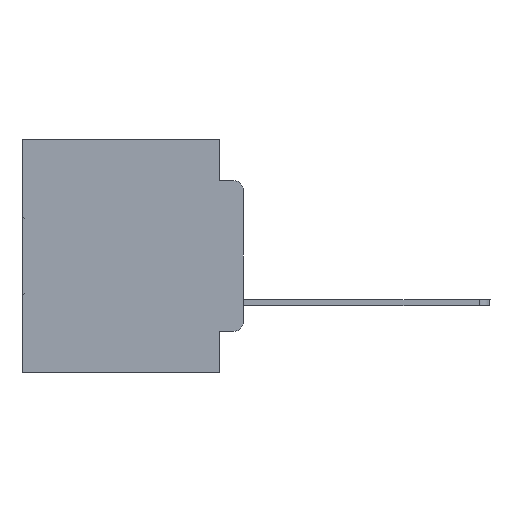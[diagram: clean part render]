
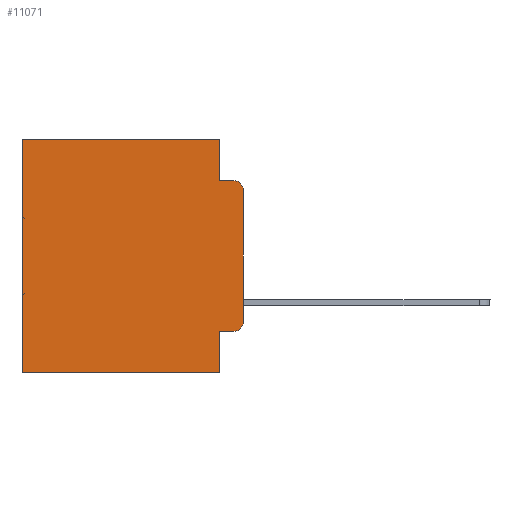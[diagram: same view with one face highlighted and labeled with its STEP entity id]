
A CAD part, left-side view. The second image highlights one B-rep face of the part: STEP entity #11071.
In plain terms, the highlighted planar face has unit normal (-1, 0, 0).
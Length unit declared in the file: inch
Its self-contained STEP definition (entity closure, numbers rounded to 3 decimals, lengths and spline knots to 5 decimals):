
#375 = CARTESIAN_POINT ( 'NONE',  ( 0.298, 0., 0. ) ) ;
#809 = CARTESIAN_POINT ( 'NONE',  ( 0.298, 0.473, 0. ) ) ;
#966 = VECTOR ( 'NONE', #11228, 39.37008 ) ;
#1144 = VERTEX_POINT ( 'NONE', #7849 ) ;
#1548 = EDGE_LOOP ( 'NONE', ( #2685, #17190, #29655, #28987, #21260, #29517, #4103, #18307, #16381, #31728 ) ) ;
#1833 = CARTESIAN_POINT ( 'NONE',  ( 0.298, 0.473, 0. ) ) ;
#1948 = LINE ( 'NONE', #13682, #32490 ) ;
#2402 = CARTESIAN_POINT ( 'NONE',  ( 0.298, 0.051, -0.4115 ) ) ;
#2685 = ORIENTED_EDGE ( 'NONE', *, *, #7705, .F. ) ;
#4091 = DIRECTION ( 'NONE',  ( -1., 0., 0. ) ) ;
#4103 = ORIENTED_EDGE ( 'NONE', *, *, #4304, .F. ) ;
#4304 = EDGE_CURVE ( 'NONE', #33011, #7289, #14189, .T. ) ;
#4448 = DIRECTION ( 'NONE',  ( 0., 0., -1. ) ) ;
#5104 = CARTESIAN_POINT ( 'NONE',  ( 0.298, 0.02, -0.3915 ) ) ;
#5167 = VERTEX_POINT ( 'NONE', #2402 ) ;
#5868 = EDGE_CURVE ( 'NONE', #33396, #25207, #22810, .T. ) ;
#6912 = CARTESIAN_POINT ( 'NONE',  ( 0.298, 0.02, -0.0885 ) ) ;
#7289 = VERTEX_POINT ( 'NONE', #31717 ) ;
#7705 = EDGE_CURVE ( 'NONE', #26355, #1144, #12773, .T. ) ;
#7849 = CARTESIAN_POINT ( 'NONE',  ( 0.298, 0., -0.3915 ) ) ;
#8508 = CARTESIAN_POINT ( 'NONE',  ( 0.298, 0., -0.1085 ) ) ;
#8758 = EDGE_CURVE ( 'NONE', #5167, #13979, #1948, .T. ) ;
#9283 = LINE ( 'NONE', #809, #966 ) ;
#9315 = AXIS2_PLACEMENT_3D ( 'NONE', #5104, #31839, #21213 ) ;
#9506 = CARTESIAN_POINT ( 'NONE',  ( 0.298, 0.051, -0.5 ) ) ;
#9947 = AXIS2_PLACEMENT_3D ( 'NONE', #23318, #17762, #4448 ) ;
#11071 = ADVANCED_FACE ( 'NONE', ( #30177 ), #20005, .F. ) ;
#11228 = DIRECTION ( 'NONE',  ( 0., 0., -1. ) ) ;
#11705 = LINE ( 'NONE', #25382, #27233 ) ;
#11950 = VECTOR ( 'NONE', #20858, 39.37008 ) ;
#12652 = CARTESIAN_POINT ( 'NONE',  ( 0.298, 0., -0.5 ) ) ;
#12773 = LINE ( 'NONE', #15342, #11950 ) ;
#13682 = CARTESIAN_POINT ( 'NONE',  ( 0.298, 0.051, -0.4115 ) ) ;
#13979 = VERTEX_POINT ( 'NONE', #15145 ) ;
#14189 = LINE ( 'NONE', #12652, #34024 ) ;
#15145 = CARTESIAN_POINT ( 'NONE',  ( 0.298, 0.02, -0.4115 ) ) ;
#15158 = VERTEX_POINT ( 'NONE', #1833 ) ;
#15244 = DIRECTION ( 'NONE',  ( 0., 0., -1. ) ) ;
#15342 = CARTESIAN_POINT ( 'NONE',  ( 0.298, 0., 0. ) ) ;
#16381 = ORIENTED_EDGE ( 'NONE', *, *, #8758, .T. ) ;
#16757 = LINE ( 'NONE', #33360, #17620 ) ;
#17190 = ORIENTED_EDGE ( 'NONE', *, *, #32377, .T. ) ;
#17305 = DIRECTION ( 'NONE',  ( 0., 0., -1. ) ) ;
#17620 = VECTOR ( 'NONE', #22855, 39.37008 ) ;
#17762 = DIRECTION ( 'NONE',  ( 1., 0., 0. ) ) ;
#18271 = EDGE_CURVE ( 'NONE', #15158, #7289, #9283, .T. ) ;
#18307 = ORIENTED_EDGE ( 'NONE', *, *, #21611, .F. ) ;
#19086 = VECTOR ( 'NONE', #15244, 39.37008 ) ;
#19415 = CARTESIAN_POINT ( 'NONE',  ( 0.298, 0.051, -0.0885 ) ) ;
#19526 = CIRCLE ( 'NONE', #28330, 0.02 ) ;
#19815 = CARTESIAN_POINT ( 'NONE',  ( 0.298, 0.02, -0.1085 ) ) ;
#20005 = PLANE ( 'NONE',  #9947 ) ;
#20367 = EDGE_CURVE ( 'NONE', #33396, #15158, #31499, .T. ) ;
#20858 = DIRECTION ( 'NONE',  ( 0., 0., -1. ) ) ;
#21213 = DIRECTION ( 'NONE',  ( 0., 0., -1. ) ) ;
#21260 = ORIENTED_EDGE ( 'NONE', *, *, #20367, .T. ) ;
#21561 = CARTESIAN_POINT ( 'NONE',  ( 0.298, 0.051, 0. ) ) ;
#21611 = EDGE_CURVE ( 'NONE', #5167, #33011, #11705, .T. ) ;
#22810 = LINE ( 'NONE', #28190, #19086 ) ;
#22855 = DIRECTION ( 'NONE',  ( 0., -1., 0. ) ) ;
#23318 = CARTESIAN_POINT ( 'NONE',  ( 0.298, 0., 0. ) ) ;
#23935 = VERTEX_POINT ( 'NONE', #6912 ) ;
#24089 = DIRECTION ( 'NONE',  ( 0., -1., 0. ) ) ;
#24184 = DIRECTION ( 'NONE',  ( 0., 1., 0. ) ) ;
#25004 = DIRECTION ( 'NONE',  ( 0., 0., -1. ) ) ;
#25207 = VERTEX_POINT ( 'NONE', #19415 ) ;
#25382 = CARTESIAN_POINT ( 'NONE',  ( 0.298, 0.051, 0. ) ) ;
#25822 = DIRECTION ( 'NONE',  ( 0., 1., 0. ) ) ;
#26355 = VERTEX_POINT ( 'NONE', #8508 ) ;
#27233 = VECTOR ( 'NONE', #17305, 39.37008 ) ;
#28190 = CARTESIAN_POINT ( 'NONE',  ( 0.298, 0.051, 0. ) ) ;
#28330 = AXIS2_PLACEMENT_3D ( 'NONE', #19815, #4091, #25004 ) ;
#28987 = ORIENTED_EDGE ( 'NONE', *, *, #5868, .F. ) ;
#29517 = ORIENTED_EDGE ( 'NONE', *, *, #18271, .T. ) ;
#29655 = ORIENTED_EDGE ( 'NONE', *, *, #30678, .F. ) ;
#30177 = FACE_OUTER_BOUND ( 'NONE', #1548, .T. ) ;
#30678 = EDGE_CURVE ( 'NONE', #25207, #23935, #16757, .T. ) ;
#31499 = LINE ( 'NONE', #375, #33161 ) ;
#31717 = CARTESIAN_POINT ( 'NONE',  ( 0.298, 0.473, -0.5 ) ) ;
#31728 = ORIENTED_EDGE ( 'NONE', *, *, #34243, .T. ) ;
#31839 = DIRECTION ( 'NONE',  ( -1., 0., 0. ) ) ;
#32377 = EDGE_CURVE ( 'NONE', #26355, #23935, #19526, .T. ) ;
#32490 = VECTOR ( 'NONE', #24089, 39.37008 ) ;
#33011 = VERTEX_POINT ( 'NONE', #9506 ) ;
#33161 = VECTOR ( 'NONE', #24184, 39.37008 ) ;
#33360 = CARTESIAN_POINT ( 'NONE',  ( 0.298, 0.051, -0.0885 ) ) ;
#33396 = VERTEX_POINT ( 'NONE', #21561 ) ;
#33438 = CIRCLE ( 'NONE', #9315, 0.02 ) ;
#34024 = VECTOR ( 'NONE', #25822, 39.37008 ) ;
#34243 = EDGE_CURVE ( 'NONE', #13979, #1144, #33438, .T. ) ;
